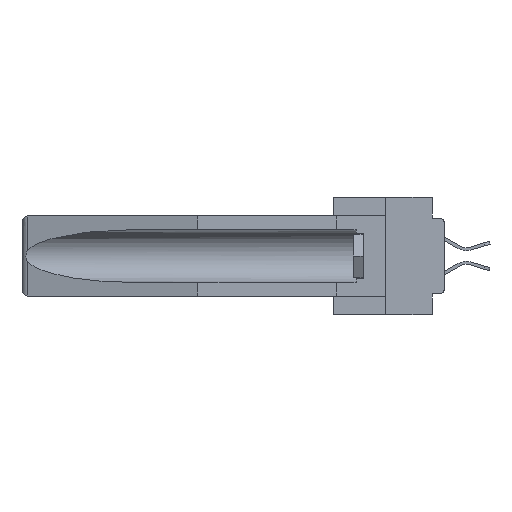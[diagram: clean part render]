
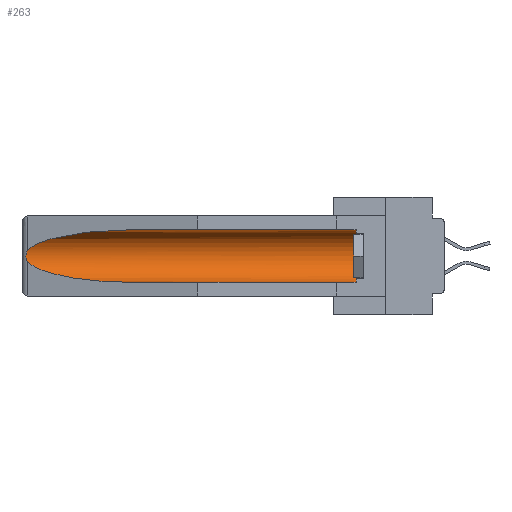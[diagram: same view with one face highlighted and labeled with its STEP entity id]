
A CAD part, left-side view. The second image highlights one B-rep face of the part: STEP entity #263.
In plain terms, the highlighted cylindrical face has radius 2.857 mm (diameter 5.715 mm), a partial arc.
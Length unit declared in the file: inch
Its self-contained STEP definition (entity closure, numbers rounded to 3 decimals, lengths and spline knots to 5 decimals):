
#81 = CARTESIAN_POINT ( 'NONE',  ( 0.26654, 1.53092, -0.15636 ) ) ;
#263 = ADVANCED_FACE ( 'NONE', ( #13067 ), #29847, .F. ) ;
#757 = VERTEX_POINT ( 'NONE', #2700 ) ;
#1685 = EDGE_CURVE ( 'NONE', #757, #3085, #18713, .T. ) ;
#1896 = DIRECTION ( 'NONE',  ( 0., 0., 1. ) ) ;
#1989 = ORIENTED_EDGE ( 'NONE', *, *, #1685, .F. ) ;
#2700 = CARTESIAN_POINT ( 'NONE',  ( 0.155, 0.126, -0.284 ) ) ;
#3021 = CARTESIAN_POINT ( 'NONE',  ( 0.25451, 1.48313, -0.24835 ) ) ;
#3085 = VERTEX_POINT ( 'NONE', #7945 ) ;
#4462 = DIRECTION ( 'NONE',  ( 0., 1., 0. ) ) ;
#5236 = CARTESIAN_POINT ( 'NONE',  ( 0.26597, 1.5296, -0.19026 ) ) ;
#5496 = DIRECTION ( 'NONE',  ( 0., 0., 1. ) ) ;
#6316 = CARTESIAN_POINT ( 'NONE',  ( 0.21114, 1.30732, -0.284 ) ) ;
#6574 = VECTOR ( 'NONE', #35869, 39.37008 ) ;
#6693 = ORIENTED_EDGE ( 'NONE', *, *, #30729, .T. ) ;
#7384 = CIRCLE ( 'NONE', #12068, 0.1125 ) ;
#7945 = CARTESIAN_POINT ( 'NONE',  ( 0.155, 1.07973, -0.284 ) ) ;
#8331 = CARTESIAN_POINT ( 'NONE',  ( 0.26537, 1.52718, -0.19328 ) ) ;
#8581 = VECTOR ( 'NONE', #23291, 39.37008 ) ;
#10654 = CARTESIAN_POINT ( 'NONE',  ( 0.155, 0.126, -0.059 ) ) ;
#10691 = CARTESIAN_POINT ( 'NONE',  ( 0.155, -0.30754, -0.284 ) ) ;
#10893 = CARTESIAN_POINT ( 'NONE',  ( 0.2673, 1.53269, -0.17917 ) ) ;
#11643 = CARTESIAN_POINT ( 'NONE',  ( 0.26537, 1.52718, -0.14972 ) ) ;
#11945 = EDGE_CURVE ( 'NONE', #34061, #12603, #32829, .T. ) ;
#12068 = AXIS2_PLACEMENT_3D ( 'NONE', #19542, #22453, #5496 ) ;
#12350 = CARTESIAN_POINT ( 'NONE',  ( 0.155, -0.30754, -0.059 ) ) ;
#12603 = VERTEX_POINT ( 'NONE', #19904 ) ;
#13067 = FACE_OUTER_BOUND ( 'NONE', #20643, .T. ) ;
#13099 = EDGE_CURVE ( 'NONE', #22206, #34061, #28585, .T. ) ;
#14758 = CARTESIAN_POINT ( 'NONE',  ( 0.25451, 1.48313, -0.09465 ) ) ;
#15798 = CARTESIAN_POINT ( 'NONE',  ( 0.155, -0.30754, -0.1715 ) ) ;
#17118 = CARTESIAN_POINT ( 'NONE',  ( 0.26537, 1.52718, -0.19328 ) ) ;
#17151 = VERTEX_POINT ( 'NONE', #8331 ) ;
#17830 = ORIENTED_EDGE ( 'NONE', *, *, #13099, .T. ) ;
#18713 = LINE ( 'NONE', #10691, #6574 ) ;
#19106 = CARTESIAN_POINT ( 'NONE',  ( 0.26537, 1.52718, -0.19328 ) ) ;
#19284 = CARTESIAN_POINT ( 'NONE',  ( 0.2673, 1.5327, -0.16383 ) ) ;
#19542 = CARTESIAN_POINT ( 'NONE',  ( 0.155, 0.126, -0.1715 ) ) ;
#19904 = CARTESIAN_POINT ( 'NONE',  ( 0.26537, 1.52718, -0.14972 ) ) ;
#20643 = EDGE_LOOP ( 'NONE', ( #27843, #34135, #26934, #1989, #6693, #17830 ) ) ;
#20974 =( BOUNDED_CURVE ( )  B_SPLINE_CURVE ( 3, ( #17118, #3021, #6316, #26010 ),
 .UNSPECIFIED., .F., .F. ) 
 B_SPLINE_CURVE_WITH_KNOTS ( ( 4, 4 ),
 ( 0.1948, 1.5708 ),
 .UNSPECIFIED. ) 
 CURVE ( )  GEOMETRIC_REPRESENTATION_ITEM ( )  RATIONAL_B_SPLINE_CURVE ( ( 1., 0.848, 0.848, 1. ) ) 
 REPRESENTATION_ITEM ( '' )  );
#22200 = CARTESIAN_POINT ( 'NONE',  ( 0.26597, 1.52961, -0.15275 ) ) ;
#22206 = VERTEX_POINT ( 'NONE', #10654 ) ;
#22453 = DIRECTION ( 'NONE',  ( 0., -1., 0. ) ) ;
#23291 = DIRECTION ( 'NONE',  ( 0., 1., 0. ) ) ;
#25118 = CARTESIAN_POINT ( 'NONE',  ( 0.26537, 1.52718, -0.14972 ) ) ;
#25666 = CARTESIAN_POINT ( 'NONE',  ( 0.21114, 1.30732, -0.059 ) ) ;
#26010 = CARTESIAN_POINT ( 'NONE',  ( 0.155, 1.07973, -0.284 ) ) ;
#26934 = ORIENTED_EDGE ( 'NONE', *, *, #27185, .T. ) ;
#27185 = EDGE_CURVE ( 'NONE', #17151, #3085, #20974, .T. ) ;
#27843 = ORIENTED_EDGE ( 'NONE', *, *, #11945, .T. ) ;
#27852 = CARTESIAN_POINT ( 'NONE',  ( 0.2675, 1.53308, -0.17534 ) ) ;
#28585 = LINE ( 'NONE', #12350, #8581 ) ;
#29086 = CARTESIAN_POINT ( 'NONE',  ( 0.155, 1.07973, -0.059 ) ) ;
#29847 = CYLINDRICAL_SURFACE ( 'NONE', #31805, 0.1125 ) ;
#30729 = EDGE_CURVE ( 'NONE', #757, #22206, #7384, .T. ) ;
#31538 = CARTESIAN_POINT ( 'NONE',  ( 0.155, 1.07973, -0.059 ) ) ;
#31805 = AXIS2_PLACEMENT_3D ( 'NONE', #15798, #4462, #1896 ) ;
#32829 =( BOUNDED_CURVE ( )  B_SPLINE_CURVE ( 3, ( #31538, #25666, #14758, #11643 ),
 .UNSPECIFIED., .F., .F. ) 
 B_SPLINE_CURVE_WITH_KNOTS ( ( 4, 4 ),
 ( 4.71239, 6.08839 ),
 .UNSPECIFIED. ) 
 CURVE ( )  GEOMETRIC_REPRESENTATION_ITEM ( )  RATIONAL_B_SPLINE_CURVE ( ( 1., 0.848, 0.848, 1. ) ) 
 REPRESENTATION_ITEM ( '' )  );
#32863 = EDGE_CURVE ( 'NONE', #12603, #17151, #34087, .T. ) ;
#34061 = VERTEX_POINT ( 'NONE', #29086 ) ;
#34087 = B_SPLINE_CURVE_WITH_KNOTS ( 'NONE', 3,
 ( #25118, #22200, #81, #19284, #35903, #27852, #10893, #36077, #5236, #19106 ),
 .UNSPECIFIED., .F., .F.,
 ( 4, 2, 2, 2, 4 ),
 ( 0., 0.00029, 0.00058, 0.00087, 0.00117 ),
 .UNSPECIFIED. ) ;
#34135 = ORIENTED_EDGE ( 'NONE', *, *, #32863, .T. ) ;
#35869 = DIRECTION ( 'NONE',  ( 0., 1., 0. ) ) ;
#35903 = CARTESIAN_POINT ( 'NONE',  ( 0.2675, 1.53308, -0.16763 ) ) ;
#36077 = CARTESIAN_POINT ( 'NONE',  ( 0.26655, 1.53094, -0.18657 ) ) ;
